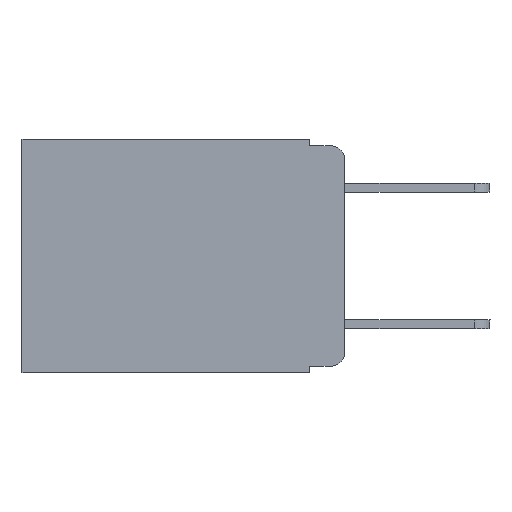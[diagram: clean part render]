
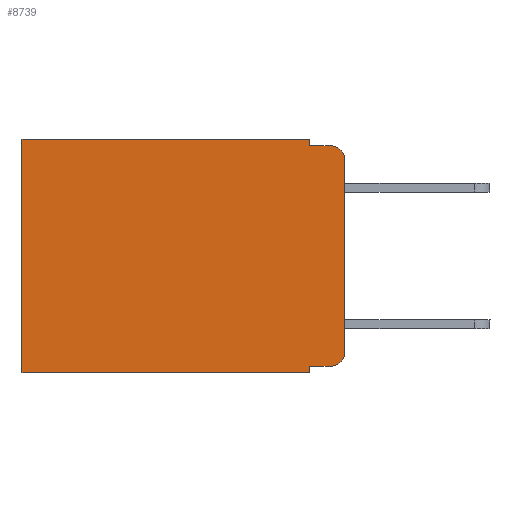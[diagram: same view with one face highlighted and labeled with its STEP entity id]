
A CAD part, left-side view. The second image highlights one B-rep face of the part: STEP entity #8739.
In plain terms, the highlighted planar face has unit normal (-1, 0, 0).
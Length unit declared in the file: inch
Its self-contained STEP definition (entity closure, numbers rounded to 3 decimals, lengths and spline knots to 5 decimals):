
#142 = VECTOR ( 'NONE', #21715, 39.37008 ) ;
#360 = EDGE_CURVE ( 'NONE', #21987, #18957, #7521, .T. ) ;
#682 = CARTESIAN_POINT ( 'NONE',  ( 0.298, 0., -0.03 ) ) ;
#702 = VECTOR ( 'NONE', #25067, 39.37008 ) ;
#1006 = EDGE_CURVE ( 'NONE', #3446, #18888, #16183, .T. ) ;
#1319 = EDGE_CURVE ( 'NONE', #25484, #18957, #4394, .T. ) ;
#1562 = ORIENTED_EDGE ( 'NONE', *, *, #1319, .T. ) ;
#1608 = DIRECTION ( 'NONE',  ( 0., 0., -1. ) ) ;
#1617 = CARTESIAN_POINT ( 'NONE',  ( 0.298, 0.051, 0. ) ) ;
#2380 = ORIENTED_EDGE ( 'NONE', *, *, #10164, .F. ) ;
#2769 = AXIS2_PLACEMENT_3D ( 'NONE', #9367, #15741, #21482 ) ;
#3446 = VERTEX_POINT ( 'NONE', #24045 ) ;
#3715 = LINE ( 'NONE', #22603, #24688 ) ;
#3977 = LINE ( 'NONE', #9258, #5194 ) ;
#3985 = PLANE ( 'NONE',  #22177 ) ;
#4394 = CIRCLE ( 'NONE', #22968, 0.02 ) ;
#4696 = CARTESIAN_POINT ( 'NONE',  ( 0.298, 0.051, 0. ) ) ;
#4933 = EDGE_CURVE ( 'NONE', #3446, #21987, #16739, .T. ) ;
#5194 = VECTOR ( 'NONE', #21379, 39.37008 ) ;
#5249 = DIRECTION ( 'NONE',  ( 0., 0., -1. ) ) ;
#5696 = CARTESIAN_POINT ( 'NONE',  ( 0.298, 0., -0.313 ) ) ;
#5982 = CARTESIAN_POINT ( 'NONE',  ( 0.298, 0.051, -0.01 ) ) ;
#6634 = CIRCLE ( 'NONE', #2769, 0.02 ) ;
#6643 = EDGE_LOOP ( 'NONE', ( #2380, #1562, #16963, #24008, #21388, #19210, #24408, #22742, #11315, #20383 ) ) ;
#7362 = DIRECTION ( 'NONE',  ( -1., 0., 0. ) ) ;
#7521 = LINE ( 'NONE', #5982, #142 ) ;
#7561 = VERTEX_POINT ( 'NONE', #10931 ) ;
#7933 = CARTESIAN_POINT ( 'NONE',  ( 0.298, 0.051, -0.333 ) ) ;
#8196 = VERTEX_POINT ( 'NONE', #8523 ) ;
#8523 = CARTESIAN_POINT ( 'NONE',  ( 0.298, 0.473, -0.343 ) ) ;
#8739 = ADVANCED_FACE ( 'NONE', ( #22988 ), #3985, .F. ) ;
#9258 = CARTESIAN_POINT ( 'NONE',  ( 0.298, 0., -0.343 ) ) ;
#9367 = CARTESIAN_POINT ( 'NONE',  ( 0.298, 0.02, -0.313 ) ) ;
#10164 = EDGE_CURVE ( 'NONE', #25484, #23553, #3715, .T. ) ;
#10776 = DIRECTION ( 'NONE',  ( 0., 0., -1. ) ) ;
#10880 = VECTOR ( 'NONE', #5249, 39.37008 ) ;
#10931 = CARTESIAN_POINT ( 'NONE',  ( 0.298, 0.02, -0.333 ) ) ;
#11315 = ORIENTED_EDGE ( 'NONE', *, *, #19421, .T. ) ;
#11919 = EDGE_CURVE ( 'NONE', #18637, #8196, #3977, .T. ) ;
#12300 = DIRECTION ( 'NONE',  ( 0., 0., -1. ) ) ;
#12354 = DIRECTION ( 'NONE',  ( 0., 0., -1. ) ) ;
#12386 = DIRECTION ( 'NONE',  ( 1., 0., 0. ) ) ;
#12426 = CARTESIAN_POINT ( 'NONE',  ( 0.298, 0.473, 0. ) ) ;
#13405 = EDGE_CURVE ( 'NONE', #7561, #23553, #6634, .T. ) ;
#13443 = CARTESIAN_POINT ( 'NONE',  ( 0.298, 0.02, -0.03 ) ) ;
#13565 = CARTESIAN_POINT ( 'NONE',  ( 0.298, 0.051, -0.01 ) ) ;
#14290 = VECTOR ( 'NONE', #19805, 39.37008 ) ;
#15012 = EDGE_CURVE ( 'NONE', #18888, #8196, #20176, .T. ) ;
#15541 = VERTEX_POINT ( 'NONE', #22649 ) ;
#15741 = DIRECTION ( 'NONE',  ( -1., 0., 0. ) ) ;
#16183 = LINE ( 'NONE', #19154, #702 ) ;
#16462 = VECTOR ( 'NONE', #17523, 39.37008 ) ;
#16739 = LINE ( 'NONE', #4696, #20715 ) ;
#16963 = ORIENTED_EDGE ( 'NONE', *, *, #360, .F. ) ;
#17523 = DIRECTION ( 'NONE',  ( 0., 0., -1. ) ) ;
#18637 = VERTEX_POINT ( 'NONE', #19236 ) ;
#18888 = VERTEX_POINT ( 'NONE', #12426 ) ;
#18957 = VERTEX_POINT ( 'NONE', #20229 ) ;
#19154 = CARTESIAN_POINT ( 'NONE',  ( 0.298, 0., 0. ) ) ;
#19210 = ORIENTED_EDGE ( 'NONE', *, *, #15012, .T. ) ;
#19236 = CARTESIAN_POINT ( 'NONE',  ( 0.298, 0.051, -0.343 ) ) ;
#19254 = LINE ( 'NONE', #1617, #16462 ) ;
#19421 = EDGE_CURVE ( 'NONE', #15541, #7561, #24791, .T. ) ;
#19805 = DIRECTION ( 'NONE',  ( 0., -1., 0. ) ) ;
#20176 = LINE ( 'NONE', #25364, #10880 ) ;
#20229 = CARTESIAN_POINT ( 'NONE',  ( 0.298, 0.02, -0.01 ) ) ;
#20368 = CARTESIAN_POINT ( 'NONE',  ( 0.298, 0., 0. ) ) ;
#20383 = ORIENTED_EDGE ( 'NONE', *, *, #13405, .T. ) ;
#20670 = EDGE_CURVE ( 'NONE', #15541, #18637, #19254, .T. ) ;
#20715 = VECTOR ( 'NONE', #12354, 39.37008 ) ;
#21379 = DIRECTION ( 'NONE',  ( 0., 1., 0. ) ) ;
#21388 = ORIENTED_EDGE ( 'NONE', *, *, #1006, .T. ) ;
#21482 = DIRECTION ( 'NONE',  ( 0., 0., -1. ) ) ;
#21715 = DIRECTION ( 'NONE',  ( 0., -1., 0. ) ) ;
#21987 = VERTEX_POINT ( 'NONE', #13565 ) ;
#22177 = AXIS2_PLACEMENT_3D ( 'NONE', #20368, #12386, #12300 ) ;
#22603 = CARTESIAN_POINT ( 'NONE',  ( 0.298, 0., 0. ) ) ;
#22649 = CARTESIAN_POINT ( 'NONE',  ( 0.298, 0.051, -0.333 ) ) ;
#22742 = ORIENTED_EDGE ( 'NONE', *, *, #20670, .F. ) ;
#22968 = AXIS2_PLACEMENT_3D ( 'NONE', #13443, #7362, #1608 ) ;
#22988 = FACE_OUTER_BOUND ( 'NONE', #6643, .T. ) ;
#23553 = VERTEX_POINT ( 'NONE', #5696 ) ;
#24008 = ORIENTED_EDGE ( 'NONE', *, *, #4933, .F. ) ;
#24045 = CARTESIAN_POINT ( 'NONE',  ( 0.298, 0.051, 0. ) ) ;
#24408 = ORIENTED_EDGE ( 'NONE', *, *, #11919, .F. ) ;
#24688 = VECTOR ( 'NONE', #10776, 39.37008 ) ;
#24791 = LINE ( 'NONE', #7933, #14290 ) ;
#25067 = DIRECTION ( 'NONE',  ( 0., 1., 0. ) ) ;
#25364 = CARTESIAN_POINT ( 'NONE',  ( 0.298, 0.473, 0. ) ) ;
#25484 = VERTEX_POINT ( 'NONE', #682 ) ;
